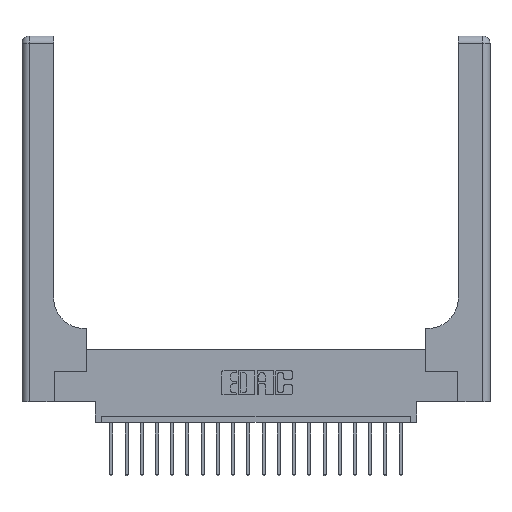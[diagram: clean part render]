
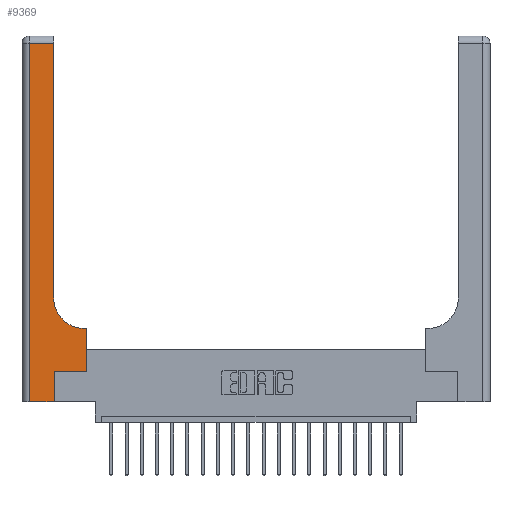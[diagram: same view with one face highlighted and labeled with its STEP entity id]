
A CAD part, top view. The second image highlights one B-rep face of the part: STEP entity #9369.
In plain terms, the highlighted planar face has unit normal (0, 0, 1).
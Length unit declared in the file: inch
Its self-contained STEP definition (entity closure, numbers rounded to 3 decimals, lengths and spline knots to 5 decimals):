
#484 = LINE ( 'NONE', #18224, #16011 ) ;
#497 = DIRECTION ( 'NONE',  ( 0., 1., 0. ) ) ;
#1652 = DIRECTION ( 'NONE',  ( -1., 0., 0. ) ) ;
#1745 = VERTEX_POINT ( 'NONE', #17420 ) ;
#1946 = EDGE_CURVE ( 'NONE', #5603, #14242, #6552, .T. ) ;
#2049 = PLANE ( 'NONE',  #2971 ) ;
#2093 = DIRECTION ( 'NONE',  ( 0., 1., 0. ) ) ;
#2122 = CARTESIAN_POINT ( 'NONE',  ( 0.26, 2.94, 0.37 ) ) ;
#2320 = EDGE_CURVE ( 'NONE', #1745, #19664, #10533, .T. ) ;
#2370 = CARTESIAN_POINT ( 'NONE',  ( 0.265, 0., 0.37 ) ) ;
#2396 = VERTEX_POINT ( 'NONE', #14895 ) ;
#2533 = CARTESIAN_POINT ( 'NONE',  ( 0.265, 0.25, 0.37 ) ) ;
#2849 = LINE ( 'NONE', #18799, #5109 ) ;
#2891 = LINE ( 'NONE', #14653, #20370 ) ;
#2910 = DIRECTION ( 'NONE',  ( -1., 0., 0. ) ) ;
#2971 = AXIS2_PLACEMENT_3D ( 'NONE', #16376, #10251, #19666 ) ;
#3285 = CARTESIAN_POINT ( 'NONE',  ( 0.528, 0.25, 0.37 ) ) ;
#3473 = DIRECTION ( 'NONE',  ( 0., 1., 0. ) ) ;
#3987 = CARTESIAN_POINT ( 'NONE',  ( 0.265, 0., 0.37 ) ) ;
#4596 = ORIENTED_EDGE ( 'NONE', *, *, #19945, .T. ) ;
#5109 = VECTOR ( 'NONE', #20371, 39.37008 ) ;
#5603 = VERTEX_POINT ( 'NONE', #14321 ) ;
#5612 = CARTESIAN_POINT ( 'NONE',  ( 0.06, 3., 0.37 ) ) ;
#5948 = EDGE_CURVE ( 'NONE', #14242, #16268, #2891, .T. ) ;
#5959 = CARTESIAN_POINT ( 'NONE',  ( 0.06, 0., 0.37 ) ) ;
#5968 = ORIENTED_EDGE ( 'NONE', *, *, #8798, .T. ) ;
#6000 = CARTESIAN_POINT ( 'NONE',  ( 0.26, 0.6, 0.37 ) ) ;
#6552 = LINE ( 'NONE', #5612, #14021 ) ;
#6584 = LINE ( 'NONE', #11643, #13570 ) ;
#6712 = LINE ( 'NONE', #11246, #20195 ) ;
#6809 = FACE_OUTER_BOUND ( 'NONE', #18858, .T. ) ;
#7082 = EDGE_CURVE ( 'NONE', #10315, #18086, #2849, .T. ) ;
#7098 = ORIENTED_EDGE ( 'NONE', *, *, #11419, .T. ) ;
#7673 = ORIENTED_EDGE ( 'NONE', *, *, #5948, .T. ) ;
#7852 = EDGE_CURVE ( 'NONE', #16268, #10315, #11921, .T. ) ;
#8798 = EDGE_CURVE ( 'NONE', #18086, #1745, #6584, .T. ) ;
#8833 = VERTEX_POINT ( 'NONE', #2122 ) ;
#9216 = ORIENTED_EDGE ( 'NONE', *, *, #7082, .T. ) ;
#9274 = ORIENTED_EDGE ( 'NONE', *, *, #2320, .T. ) ;
#9369 = ADVANCED_FACE ( 'NONE', ( #6809 ), #2049, .F. ) ;
#9864 = ORIENTED_EDGE ( 'NONE', *, *, #7852, .T. ) ;
#9968 = AXIS2_PLACEMENT_3D ( 'NONE', #10053, #19425, #17874 ) ;
#9981 = DIRECTION ( 'NONE',  ( 1., 0., 0. ) ) ;
#10053 = CARTESIAN_POINT ( 'NONE',  ( 0.51, 0.85, 0.37 ) ) ;
#10251 = DIRECTION ( 'NONE',  ( 0., 0., -1. ) ) ;
#10315 = VERTEX_POINT ( 'NONE', #2533 ) ;
#10533 = LINE ( 'NONE', #6000, #13284 ) ;
#11246 = CARTESIAN_POINT ( 'NONE',  ( 0., 2.94, 0.37 ) ) ;
#11419 = EDGE_CURVE ( 'NONE', #8833, #5603, #6712, .T. ) ;
#11643 = CARTESIAN_POINT ( 'NONE',  ( 0.528, 0.25, 0.37 ) ) ;
#11921 = LINE ( 'NONE', #2370, #13895 ) ;
#13188 = ORIENTED_EDGE ( 'NONE', *, *, #1946, .T. ) ;
#13284 = VECTOR ( 'NONE', #2910, 39.37008 ) ;
#13570 = VECTOR ( 'NONE', #497, 39.37008 ) ;
#13895 = VECTOR ( 'NONE', #2093, 39.37008 ) ;
#14021 = VECTOR ( 'NONE', #15021, 39.37008 ) ;
#14242 = VERTEX_POINT ( 'NONE', #5959 ) ;
#14321 = CARTESIAN_POINT ( 'NONE',  ( 0.06, 2.94, 0.37 ) ) ;
#14653 = CARTESIAN_POINT ( 'NONE',  ( 0., 0., 0.37 ) ) ;
#14895 = CARTESIAN_POINT ( 'NONE',  ( 0.26, 0.85, 0.37 ) ) ;
#15021 = DIRECTION ( 'NONE',  ( 0., -1., 0. ) ) ;
#16011 = VECTOR ( 'NONE', #3473, 39.37008 ) ;
#16268 = VERTEX_POINT ( 'NONE', #3987 ) ;
#16376 = CARTESIAN_POINT ( 'NONE',  ( 0., 3., 0.37 ) ) ;
#17278 = ORIENTED_EDGE ( 'NONE', *, *, #18624, .T. ) ;
#17420 = CARTESIAN_POINT ( 'NONE',  ( 0.528, 0.6, 0.37 ) ) ;
#17874 = DIRECTION ( 'NONE',  ( 1., 0., 0. ) ) ;
#18086 = VERTEX_POINT ( 'NONE', #3285 ) ;
#18224 = CARTESIAN_POINT ( 'NONE',  ( 0.26, 3., 0.37 ) ) ;
#18624 = EDGE_CURVE ( 'NONE', #2396, #8833, #484, .T. ) ;
#18738 = CARTESIAN_POINT ( 'NONE',  ( 0.51, 0.6, 0.37 ) ) ;
#18799 = CARTESIAN_POINT ( 'NONE',  ( 0.265, 0.25, 0.37 ) ) ;
#18858 = EDGE_LOOP ( 'NONE', ( #17278, #7098, #13188, #7673, #9864, #9216, #5968, #9274, #4596 ) ) ;
#19425 = DIRECTION ( 'NONE',  ( 0., 0., -1. ) ) ;
#19463 = CIRCLE ( 'NONE', #9968, 0.25 ) ;
#19664 = VERTEX_POINT ( 'NONE', #18738 ) ;
#19666 = DIRECTION ( 'NONE',  ( -1., 0., 0. ) ) ;
#19945 = EDGE_CURVE ( 'NONE', #19664, #2396, #19463, .T. ) ;
#20195 = VECTOR ( 'NONE', #1652, 39.37008 ) ;
#20370 = VECTOR ( 'NONE', #9981, 39.37008 ) ;
#20371 = DIRECTION ( 'NONE',  ( 1., 0., 0. ) ) ;
